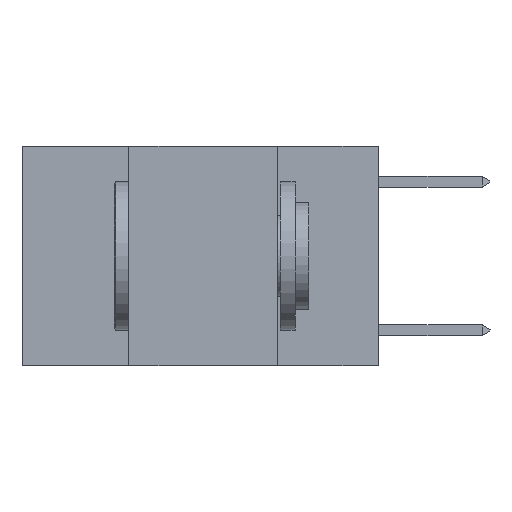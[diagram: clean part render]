
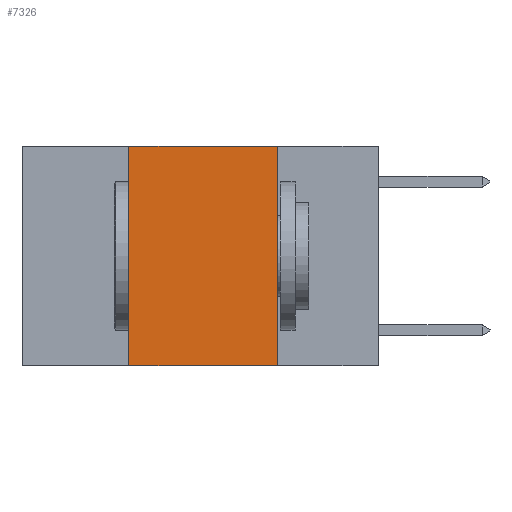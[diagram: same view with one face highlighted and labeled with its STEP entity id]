
A CAD part, left-side view. The second image highlights one B-rep face of the part: STEP entity #7326.
In plain terms, the highlighted planar face has unit normal (-1, 0, 0).
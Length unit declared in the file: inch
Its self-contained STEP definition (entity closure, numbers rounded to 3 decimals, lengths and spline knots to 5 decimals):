
#147 = DIRECTION ( 'NONE',  ( 0., -1., 0. ) ) ;
#175 = CARTESIAN_POINT ( 'NONE',  ( 0., 0.6, 0. ) ) ;
#391 = CARTESIAN_POINT ( 'NONE',  ( 0., 0.42, 0. ) ) ;
#520 = LINE ( 'NONE', #19572, #596 ) ;
#596 = VECTOR ( 'NONE', #18994, 39.37008 ) ;
#691 = VECTOR ( 'NONE', #4155, 39.37008 ) ;
#784 = EDGE_CURVE ( 'NONE', #796, #15060, #4277, .T. ) ;
#796 = VERTEX_POINT ( 'NONE', #391 ) ;
#804 = LINE ( 'NONE', #13784, #5333 ) ;
#813 = LINE ( 'NONE', #6480, #691 ) ;
#1349 = EDGE_CURVE ( 'NONE', #15060, #17540, #813, .T. ) ;
#3076 = FACE_OUTER_BOUND ( 'NONE', #11155, .T. ) ;
#4155 = DIRECTION ( 'NONE',  ( 0., 0., -1. ) ) ;
#4216 = VECTOR ( 'NONE', #147, 39.37008 ) ;
#4277 = LINE ( 'NONE', #175, #4216 ) ;
#5203 = CARTESIAN_POINT ( 'NONE',  ( 0., 0.17, 0. ) ) ;
#5333 = VECTOR ( 'NONE', #23183, 39.37008 ) ;
#6480 = CARTESIAN_POINT ( 'NONE',  ( 0., 0.17, 0. ) ) ;
#6691 = AXIS2_PLACEMENT_3D ( 'NONE', #10654, #10629, #10608 ) ;
#6749 = EDGE_CURVE ( 'NONE', #7552, #796, #520, .T. ) ;
#7326 = ADVANCED_FACE ( 'NONE', ( #3076 ), #10778, .F. ) ;
#7552 = VERTEX_POINT ( 'NONE', #7658 ) ;
#7658 = CARTESIAN_POINT ( 'NONE',  ( 0., 0.42, -0.37 ) ) ;
#10608 = DIRECTION ( 'NONE',  ( 0., 0., -1. ) ) ;
#10629 = DIRECTION ( 'NONE',  ( 1., 0., 0. ) ) ;
#10654 = CARTESIAN_POINT ( 'NONE',  ( 0., 0.6, 0. ) ) ;
#10778 = PLANE ( 'NONE',  #6691 ) ;
#11155 = EDGE_LOOP ( 'NONE', ( #11873, #12229, #12278, #12797 ) ) ;
#11873 = ORIENTED_EDGE ( 'NONE', *, *, #1349, .F. ) ;
#12229 = ORIENTED_EDGE ( 'NONE', *, *, #784, .F. ) ;
#12278 = ORIENTED_EDGE ( 'NONE', *, *, #6749, .F. ) ;
#12797 = ORIENTED_EDGE ( 'NONE', *, *, #13497, .T. ) ;
#13497 = EDGE_CURVE ( 'NONE', #7552, #17540, #804, .T. ) ;
#13784 = CARTESIAN_POINT ( 'NONE',  ( 0., 0.6, -0.37 ) ) ;
#15060 = VERTEX_POINT ( 'NONE', #5203 ) ;
#17540 = VERTEX_POINT ( 'NONE', #20443 ) ;
#18994 = DIRECTION ( 'NONE',  ( 0., 0., 1. ) ) ;
#19572 = CARTESIAN_POINT ( 'NONE',  ( 0., 0.42, 0. ) ) ;
#20443 = CARTESIAN_POINT ( 'NONE',  ( 0., 0.17, -0.37 ) ) ;
#23183 = DIRECTION ( 'NONE',  ( 0., -1., 0. ) ) ;
